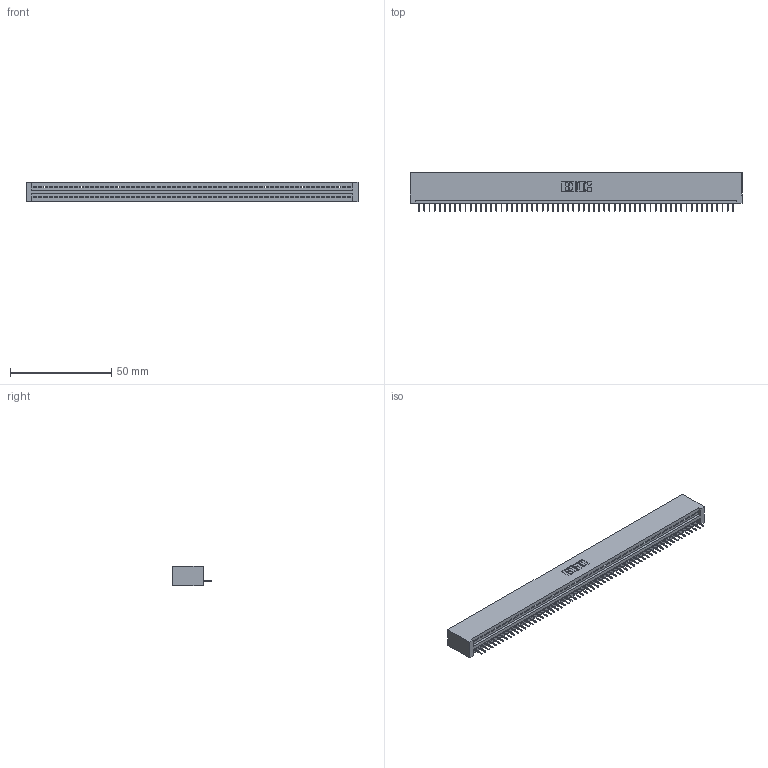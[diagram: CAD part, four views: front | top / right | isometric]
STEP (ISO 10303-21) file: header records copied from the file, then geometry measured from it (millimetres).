
FILE_DESCRIPTION (( 'STEP AP203' ), '1' );
FILE_NAME ('345-062-524-101.STEP', '2019-10-11T05:41:03', ( '' ), ( '' ), 'SwSTEP 2.0', 'SolidWorks 2016', '' );
FILE_SCHEMA (( 'CONFIG_CONTROL_DESIGN' ));
Length unit declared in the file: inch
Products named in the file (3): 345-292-001_345-293-124; 345-062-524-101; 345 Part_No Mounting Lugs
Assembly tree (63 placements, depth 2):
  345-062-524-101
    345 Part_No Mounting Lugs
    345-292-001_345-293-124  x62
Bounding box: 164.08 x 19.35 x 9.4 mm (x, y, z)
Volume: 16088.1 mm3; surface area: 21058.6 mm2
Topology: 63 solids, 63 shells, 3962 faces, 11477 edges, 7402 vertices
Faces by surface type: plane 2928, cylinder 1034
Entity records: 43767 total; most frequent: CARTESIAN_POINT 7586, ORIENTED_EDGE 7582, DIRECTION 6591, EDGE_CURVE 3791, VECTOR 3423, LINE 3423, VERTEX_POINT 2522, AXIS2_PLACEMENT_3D 1584
